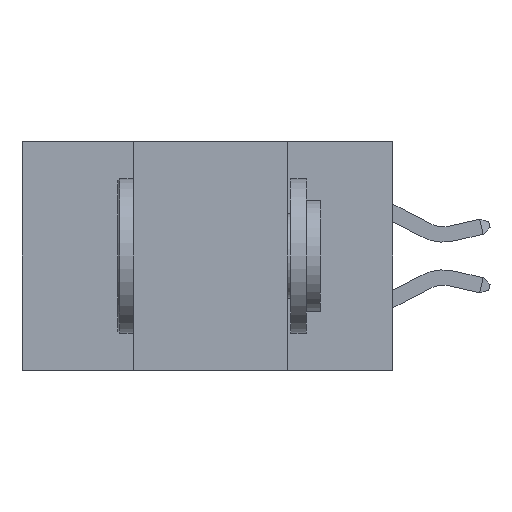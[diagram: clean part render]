
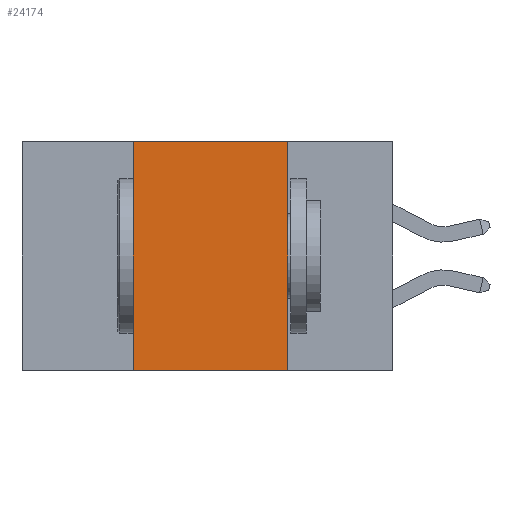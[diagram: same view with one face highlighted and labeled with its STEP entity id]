
A CAD part, left-side view. The second image highlights one B-rep face of the part: STEP entity #24174.
In plain terms, the highlighted planar face has unit normal (-1, 0, 0).
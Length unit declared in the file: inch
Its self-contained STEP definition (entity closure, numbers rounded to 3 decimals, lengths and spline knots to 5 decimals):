
#40 = DIRECTION ( 'NONE',  ( 0., -1., 0. ) ) ;
#788 = CARTESIAN_POINT ( 'NONE',  ( 0., 0.17, -0.37 ) ) ;
#1533 = EDGE_CURVE ( 'NONE', #23835, #21433, #18090, .T. ) ;
#3349 = VERTEX_POINT ( 'NONE', #788 ) ;
#3452 = CARTESIAN_POINT ( 'NONE',  ( 0., 0.17, 0. ) ) ;
#4552 = DIRECTION ( 'NONE',  ( 0., 0., -1. ) ) ;
#4831 = FACE_OUTER_BOUND ( 'NONE', #14078, .T. ) ;
#6862 = AXIS2_PLACEMENT_3D ( 'NONE', #14706, #16731, #4552 ) ;
#8658 = EDGE_CURVE ( 'NONE', #23835, #3349, #19544, .T. ) ;
#9702 = VERTEX_POINT ( 'NONE', #3452 ) ;
#10498 = DIRECTION ( 'NONE',  ( 0., 0., 1. ) ) ;
#10564 = PLANE ( 'NONE',  #6862 ) ;
#10733 = CARTESIAN_POINT ( 'NONE',  ( 0., 0.42, 0. ) ) ;
#11259 = VECTOR ( 'NONE', #25088, 39.37008 ) ;
#12926 = EDGE_CURVE ( 'NONE', #21433, #9702, #24949, .T. ) ;
#13540 = CARTESIAN_POINT ( 'NONE',  ( 0., 0.42, -0.37 ) ) ;
#13639 = VECTOR ( 'NONE', #40, 39.37008 ) ;
#14078 = EDGE_LOOP ( 'NONE', ( #23109, #19408, #21594, #18692 ) ) ;
#14153 = VECTOR ( 'NONE', #20478, 39.37008 ) ;
#14706 = CARTESIAN_POINT ( 'NONE',  ( 0., 0.6, 0. ) ) ;
#16704 = LINE ( 'NONE', #21150, #11259 ) ;
#16731 = DIRECTION ( 'NONE',  ( 1., 0., 0. ) ) ;
#17073 = CARTESIAN_POINT ( 'NONE',  ( 0., 0.42, 0. ) ) ;
#18090 = LINE ( 'NONE', #17073, #23448 ) ;
#18662 = EDGE_CURVE ( 'NONE', #9702, #3349, #16704, .T. ) ;
#18692 = ORIENTED_EDGE ( 'NONE', *, *, #8658, .T. ) ;
#19408 = ORIENTED_EDGE ( 'NONE', *, *, #12926, .F. ) ;
#19544 = LINE ( 'NONE', #24482, #14153 ) ;
#20387 = CARTESIAN_POINT ( 'NONE',  ( 0., 0.6, 0. ) ) ;
#20478 = DIRECTION ( 'NONE',  ( 0., -1., 0. ) ) ;
#21150 = CARTESIAN_POINT ( 'NONE',  ( 0., 0.17, 0. ) ) ;
#21433 = VERTEX_POINT ( 'NONE', #10733 ) ;
#21594 = ORIENTED_EDGE ( 'NONE', *, *, #1533, .F. ) ;
#23109 = ORIENTED_EDGE ( 'NONE', *, *, #18662, .F. ) ;
#23448 = VECTOR ( 'NONE', #10498, 39.37008 ) ;
#23835 = VERTEX_POINT ( 'NONE', #13540 ) ;
#24174 = ADVANCED_FACE ( 'NONE', ( #4831 ), #10564, .F. ) ;
#24482 = CARTESIAN_POINT ( 'NONE',  ( 0., 0.6, -0.37 ) ) ;
#24949 = LINE ( 'NONE', #20387, #13639 ) ;
#25088 = DIRECTION ( 'NONE',  ( 0., 0., -1. ) ) ;
